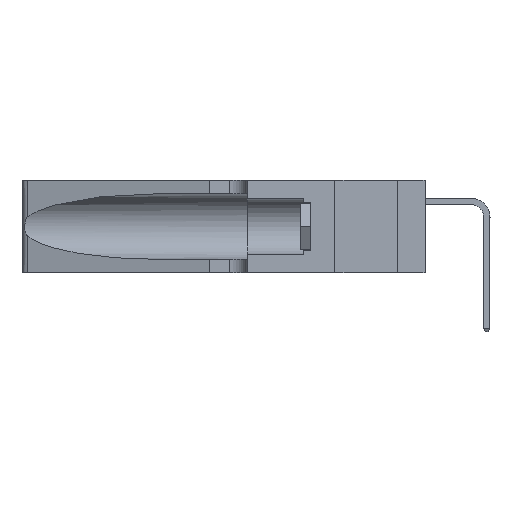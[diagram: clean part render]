
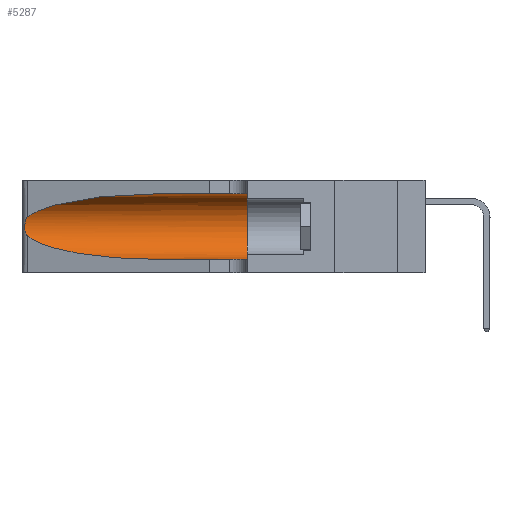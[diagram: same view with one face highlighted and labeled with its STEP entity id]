
A CAD part, left-side view. The second image highlights one B-rep face of the part: STEP entity #5287.
In plain terms, the highlighted cylindrical face has radius 3.308 mm (diameter 6.617 mm), a partial arc.
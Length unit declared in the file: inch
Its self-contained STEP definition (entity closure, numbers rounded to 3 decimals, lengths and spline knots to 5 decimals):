
#715 = DIRECTION ( 'NONE',  ( 0., -1., 0. ) ) ;
#786 = CARTESIAN_POINT ( 'NONE',  ( 0.25487, 1.22718, 0.22369 ) ) ;
#1170 = VERTEX_POINT ( 'NONE', #11796 ) ;
#1432 = ORIENTED_EDGE ( 'NONE', *, *, #26534, .T. ) ;
#1563 = DIRECTION ( 'NONE',  ( 0., 0., 1. ) ) ;
#2410 = VERTEX_POINT ( 'NONE', #22592 ) ;
#2876 = CARTESIAN_POINT ( 'NONE',  ( 0.25854, 1.2359, 0.20912 ) ) ;
#5046 = CARTESIAN_POINT ( 'NONE',  ( 0.18966, 0.96281, 0.05475 ) ) ;
#5117 = EDGE_CURVE ( 'NONE', #2410, #10378, #21428, .T. ) ;
#5287 = ADVANCED_FACE ( 'NONE', ( #12892 ), #19879, .F. ) ;
#5974 = CARTESIAN_POINT ( 'NONE',  ( 0.26075, 1.23896, 0.19203 ) ) ;
#7844 = LINE ( 'NONE', #36353, #22686 ) ;
#8807 = CARTESIAN_POINT ( 'NONE',  ( 0.25555, 1.22994, 0.2215 ) ) ;
#8919 = DIRECTION ( 'NONE',  ( 0., 0., -1. ) ) ;
#9051 = CARTESIAN_POINT ( 'NONE',  ( 0.26017, 1.23833, 0.17102 ) ) ;
#9175 = CARTESIAN_POINT ( 'NONE',  ( 0.1305, 0.72297, 0.31525 ) ) ;
#10121 = ORIENTED_EDGE ( 'NONE', *, *, #24547, .T. ) ;
#10378 = VERTEX_POINT ( 'NONE', #26470 ) ;
#11095 = ORIENTED_EDGE ( 'NONE', *, *, #33867, .F. ) ;
#11796 = CARTESIAN_POINT ( 'NONE',  ( 0.1305, 0.35, 0.31525 ) ) ;
#11891 = DIRECTION ( 'NONE',  ( 0., -1., 0. ) ) ;
#11899 = CARTESIAN_POINT ( 'NONE',  ( 0.25487, 1.22718, 0.22369 ) ) ;
#12024 = CARTESIAN_POINT ( 'NONE',  ( 0.25789, 1.23486, 0.15765 ) ) ;
#12675 = CARTESIAN_POINT ( 'NONE',  ( 0.18966, 0.96281, 0.31525 ) ) ;
#12892 = FACE_OUTER_BOUND ( 'NONE', #26375, .T. ) ;
#15008 = CARTESIAN_POINT ( 'NONE',  ( 0.25555, 1.22993, 0.14849 ) ) ;
#15663 = CARTESIAN_POINT ( 'NONE',  ( 0.25487, 1.22718, 0.22369 ) ) ;
#16187 = CIRCLE ( 'NONE', #23771, 0.13025 ) ;
#16496 = ORIENTED_EDGE ( 'NONE', *, *, #33675, .T. ) ;
#16604 = ORIENTED_EDGE ( 'NONE', *, *, #34378, .F. ) ;
#16982 = CARTESIAN_POINT ( 'NONE',  ( 0.2373, 1.15595, 0.08982 ) ) ;
#18532 = CARTESIAN_POINT ( 'NONE',  ( 0.1305, 0.72297, 0.31525 ) ) ;
#19564 = DIRECTION ( 'NONE',  ( 0., 1., 0. ) ) ;
#19830 = VERTEX_POINT ( 'NONE', #20878 ) ;
#19879 = CYLINDRICAL_SURFACE ( 'NONE', #38030, 0.13025 ) ;
#20543 = VERTEX_POINT ( 'NONE', #9175 ) ;
#20844 = CARTESIAN_POINT ( 'NONE',  ( 0.25787, 1.23484, 0.2124 ) ) ;
#20878 = CARTESIAN_POINT ( 'NONE',  ( 0.1305, 0.35, 0.05475 ) ) ;
#20977 = CARTESIAN_POINT ( 'NONE',  ( 0.1305, 1.61858, 0.05475 ) ) ;
#21229 = VECTOR ( 'NONE', #32812, 39.37008 ) ;
#21428 =( BOUNDED_CURVE ( )  B_SPLINE_CURVE ( 3, ( #37548, #16982, #5046, #25904 ),
 .UNSPECIFIED., .F., .F. ) 
 B_SPLINE_CURVE_WITH_KNOTS ( ( 4, 4 ),
 ( 3.44316, 4.71239 ),
 .UNSPECIFIED. ) 
 CURVE ( )  GEOMETRIC_REPRESENTATION_ITEM ( )  RATIONAL_B_SPLINE_CURVE ( ( 1., 0.87, 0.87, 1. ) ) 
 REPRESENTATION_ITEM ( '' )  );
#22592 = CARTESIAN_POINT ( 'NONE',  ( 0.25487, 1.22718, 0.14631 ) ) ;
#22686 = VECTOR ( 'NONE', #715, 39.37008 ) ;
#23771 = AXIS2_PLACEMENT_3D ( 'NONE', #37160, #19564, #1563 ) ;
#23816 = CARTESIAN_POINT ( 'NONE',  ( 0.26018, 1.23835, 0.19895 ) ) ;
#24118 = VERTEX_POINT ( 'NONE', #786 ) ;
#24547 = EDGE_CURVE ( 'NONE', #24118, #2410, #30877, .T. ) ;
#25904 = CARTESIAN_POINT ( 'NONE',  ( 0.1305, 0.72297, 0.05475 ) ) ;
#26375 = EDGE_LOOP ( 'NONE', ( #16496, #10121, #28757, #1432, #11095, #16604 ) ) ;
#26470 = CARTESIAN_POINT ( 'NONE',  ( 0.1305, 0.72297, 0.05475 ) ) ;
#26534 = EDGE_CURVE ( 'NONE', #10378, #19830, #30903, .T. ) ;
#26779 = CARTESIAN_POINT ( 'NONE',  ( 0.26075, 1.23896, 0.178 ) ) ;
#28757 = ORIENTED_EDGE ( 'NONE', *, *, #5117, .T. ) ;
#29714 = CARTESIAN_POINT ( 'NONE',  ( 0.25856, 1.23593, 0.16098 ) ) ;
#30877 = B_SPLINE_CURVE_WITH_KNOTS ( 'NONE', 3,
 ( #11899, #8807, #38425, #20844, #2876, #23816, #5974, #26779, #9051, #29714, #12024, #32669, #15008, #35615 ),
 .UNSPECIFIED., .F., .F.,
 ( 4, 2, 2, 2, 2, 2, 4 ),
 ( 0., 0.00027, 0.00053, 0.00107, 0.0016, 0.00187, 0.00214 ),
 .UNSPECIFIED. ) ;
#30903 = LINE ( 'NONE', #20977, #21229 ) ;
#32054 =( BOUNDED_CURVE ( )  B_SPLINE_CURVE ( 3, ( #18532, #12675, #33316, #15663 ),
 .UNSPECIFIED., .F., .T. ) 
 B_SPLINE_CURVE_WITH_KNOTS ( ( 4, 4 ),
 ( 1.5708, 2.84003 ),
 .UNSPECIFIED. ) 
 CURVE ( )  GEOMETRIC_REPRESENTATION_ITEM ( )  RATIONAL_B_SPLINE_CURVE ( ( 1., 0.87, 0.87, 1. ) ) 
 REPRESENTATION_ITEM ( '' )  );
#32539 = CARTESIAN_POINT ( 'NONE',  ( 0.1305, 1.61858, 0.185 ) ) ;
#32669 = CARTESIAN_POINT ( 'NONE',  ( 0.25639, 1.23186, 0.15144 ) ) ;
#32812 = DIRECTION ( 'NONE',  ( 0., -1., 0. ) ) ;
#33316 = CARTESIAN_POINT ( 'NONE',  ( 0.2373, 1.15595, 0.28018 ) ) ;
#33675 = EDGE_CURVE ( 'NONE', #20543, #24118, #32054, .T. ) ;
#33867 = EDGE_CURVE ( 'NONE', #1170, #19830, #16187, .T. ) ;
#34378 = EDGE_CURVE ( 'NONE', #20543, #1170, #7844, .T. ) ;
#35615 = CARTESIAN_POINT ( 'NONE',  ( 0.25487, 1.22718, 0.14631 ) ) ;
#36353 = CARTESIAN_POINT ( 'NONE',  ( 0.1305, 1.61858, 0.31525 ) ) ;
#37160 = CARTESIAN_POINT ( 'NONE',  ( 0.1305, 0.35, 0.185 ) ) ;
#37548 = CARTESIAN_POINT ( 'NONE',  ( 0.25487, 1.22718, 0.14631 ) ) ;
#38030 = AXIS2_PLACEMENT_3D ( 'NONE', #32539, #11891, #8919 ) ;
#38425 = CARTESIAN_POINT ( 'NONE',  ( 0.25639, 1.23184, 0.21858 ) ) ;
